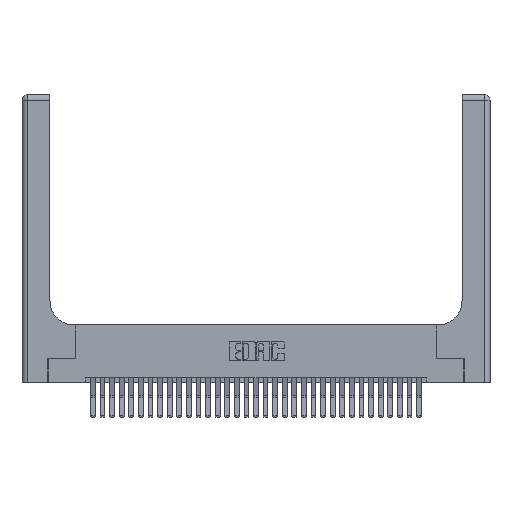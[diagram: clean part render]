
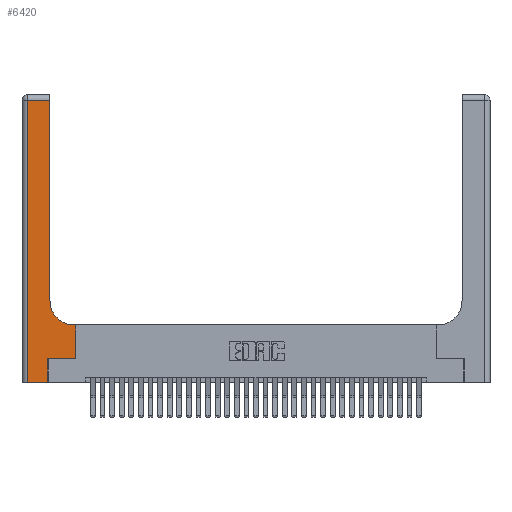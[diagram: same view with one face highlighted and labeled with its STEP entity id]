
A CAD part, top view. The second image highlights one B-rep face of the part: STEP entity #6420.
In plain terms, the highlighted planar face has unit normal (0, 0, 1).
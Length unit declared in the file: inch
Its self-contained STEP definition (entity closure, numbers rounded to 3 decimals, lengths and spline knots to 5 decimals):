
#396 = CARTESIAN_POINT ( 'NONE',  ( 0., 2.94, 0.37 ) ) ;
#876 = CARTESIAN_POINT ( 'NONE',  ( 0.2915, 0.6, 0.37 ) ) ;
#1015 = EDGE_LOOP ( 'NONE', ( #20547, #8711, #9141, #16488, #2860, #24178, #11460, #17182, #23812 ) ) ;
#1148 = CARTESIAN_POINT ( 'NONE',  ( 0.2915, 0.85, 0.37 ) ) ;
#1270 = EDGE_CURVE ( 'NONE', #16733, #8135, #19884, .T. ) ;
#1739 = CARTESIAN_POINT ( 'NONE',  ( 0.2915, 3., 0.37 ) ) ;
#1997 = CARTESIAN_POINT ( 'NONE',  ( 0.2915, 2.94, 0.37 ) ) ;
#2293 = VECTOR ( 'NONE', #3494, 39.37008 ) ;
#2794 = VECTOR ( 'NONE', #21334, 39.37008 ) ;
#2852 = LINE ( 'NONE', #9626, #32170 ) ;
#2860 = ORIENTED_EDGE ( 'NONE', *, *, #19031, .T. ) ;
#3111 = LINE ( 'NONE', #876, #2293 ) ;
#3238 = CARTESIAN_POINT ( 'NONE',  ( 0., 3., 0.37 ) ) ;
#3291 = FACE_OUTER_BOUND ( 'NONE', #1015, .T. ) ;
#3494 = DIRECTION ( 'NONE',  ( -1., 0., 0. ) ) ;
#4612 = CARTESIAN_POINT ( 'NONE',  ( 0.269, 0.25, 0.37 ) ) ;
#5867 = DIRECTION ( 'NONE',  ( -1., 0., 0. ) ) ;
#5986 = CARTESIAN_POINT ( 'NONE',  ( 0.06, 3., 0.37 ) ) ;
#6420 = ADVANCED_FACE ( 'NONE', ( #3291 ), #18890, .F. ) ;
#6477 = CARTESIAN_POINT ( 'NONE',  ( 0.5415, 0.85, 0.37 ) ) ;
#7149 = VERTEX_POINT ( 'NONE', #19201 ) ;
#7297 = VERTEX_POINT ( 'NONE', #25047 ) ;
#7369 = CARTESIAN_POINT ( 'NONE',  ( 0.06, 2.94, 0.37 ) ) ;
#8135 = VERTEX_POINT ( 'NONE', #1997 ) ;
#8263 = AXIS2_PLACEMENT_3D ( 'NONE', #6477, #24780, #9119 ) ;
#8711 = ORIENTED_EDGE ( 'NONE', *, *, #9778, .T. ) ;
#8777 = LINE ( 'NONE', #5986, #22686 ) ;
#9119 = DIRECTION ( 'NONE',  ( 1., 0., 0. ) ) ;
#9141 = ORIENTED_EDGE ( 'NONE', *, *, #18527, .T. ) ;
#9626 = CARTESIAN_POINT ( 'NONE',  ( 0.269, 0.25, 0.37 ) ) ;
#9778 = EDGE_CURVE ( 'NONE', #8135, #10173, #15036, .T. ) ;
#10173 = VERTEX_POINT ( 'NONE', #7369 ) ;
#10975 = CARTESIAN_POINT ( 'NONE',  ( 0.5585, 0.25, 0.37 ) ) ;
#10999 = DIRECTION ( 'NONE',  ( 1., 0., 0. ) ) ;
#11460 = ORIENTED_EDGE ( 'NONE', *, *, #33110, .T. ) ;
#11610 = CARTESIAN_POINT ( 'NONE',  ( 0.5585, 0.6, 0.37 ) ) ;
#11803 = EDGE_CURVE ( 'NONE', #7149, #11942, #18235, .T. ) ;
#11942 = VERTEX_POINT ( 'NONE', #13962 ) ;
#12895 = VECTOR ( 'NONE', #25295, 39.37008 ) ;
#13962 = CARTESIAN_POINT ( 'NONE',  ( 0.269, 0., 0.37 ) ) ;
#14016 = VECTOR ( 'NONE', #18294, 39.37008 ) ;
#14393 = AXIS2_PLACEMENT_3D ( 'NONE', #3238, #21555, #5867 ) ;
#14828 = LINE ( 'NONE', #15660, #14016 ) ;
#15036 = LINE ( 'NONE', #396, #2794 ) ;
#15660 = CARTESIAN_POINT ( 'NONE',  ( 0.269, 0., 0.37 ) ) ;
#16488 = ORIENTED_EDGE ( 'NONE', *, *, #11803, .T. ) ;
#16733 = VERTEX_POINT ( 'NONE', #1148 ) ;
#17182 = ORIENTED_EDGE ( 'NONE', *, *, #17292, .T. ) ;
#17292 = EDGE_CURVE ( 'NONE', #32045, #7297, #3111, .T. ) ;
#17388 = EDGE_CURVE ( 'NONE', #7297, #16733, #27611, .T. ) ;
#18235 = LINE ( 'NONE', #26665, #25216 ) ;
#18294 = DIRECTION ( 'NONE',  ( 0., 1., 0. ) ) ;
#18527 = EDGE_CURVE ( 'NONE', #10173, #7149, #8777, .T. ) ;
#18890 = PLANE ( 'NONE',  #14393 ) ;
#19031 = EDGE_CURVE ( 'NONE', #11942, #20616, #14828, .T. ) ;
#19201 = CARTESIAN_POINT ( 'NONE',  ( 0.06, 0., 0.37 ) ) ;
#19884 = LINE ( 'NONE', #1739, #12895 ) ;
#20547 = ORIENTED_EDGE ( 'NONE', *, *, #1270, .T. ) ;
#20616 = VERTEX_POINT ( 'NONE', #4612 ) ;
#21334 = DIRECTION ( 'NONE',  ( -1., 0., 0. ) ) ;
#21555 = DIRECTION ( 'NONE',  ( 0., 0., -1. ) ) ;
#22686 = VECTOR ( 'NONE', #24312, 39.37008 ) ;
#23137 = VECTOR ( 'NONE', #30707, 39.37008 ) ;
#23812 = ORIENTED_EDGE ( 'NONE', *, *, #17388, .T. ) ;
#24178 = ORIENTED_EDGE ( 'NONE', *, *, #25339, .T. ) ;
#24312 = DIRECTION ( 'NONE',  ( 0., -1., 0. ) ) ;
#24780 = DIRECTION ( 'NONE',  ( 0., 0., -1. ) ) ;
#25047 = CARTESIAN_POINT ( 'NONE',  ( 0.5415, 0.6, 0.37 ) ) ;
#25216 = VECTOR ( 'NONE', #10999, 39.37008 ) ;
#25295 = DIRECTION ( 'NONE',  ( 0., 1., 0. ) ) ;
#25339 = EDGE_CURVE ( 'NONE', #20616, #31250, #2852, .T. ) ;
#25546 = CARTESIAN_POINT ( 'NONE',  ( 0.5585, 0.25, 0.37 ) ) ;
#26665 = CARTESIAN_POINT ( 'NONE',  ( 0., 0., 0.37 ) ) ;
#27611 = CIRCLE ( 'NONE', #8263, 0.25 ) ;
#27871 = DIRECTION ( 'NONE',  ( 1., 0., 0. ) ) ;
#30707 = DIRECTION ( 'NONE',  ( 0., 1., 0. ) ) ;
#30774 = LINE ( 'NONE', #25546, #23137 ) ;
#31250 = VERTEX_POINT ( 'NONE', #10975 ) ;
#32045 = VERTEX_POINT ( 'NONE', #11610 ) ;
#32170 = VECTOR ( 'NONE', #27871, 39.37008 ) ;
#33110 = EDGE_CURVE ( 'NONE', #31250, #32045, #30774, .T. ) ;
